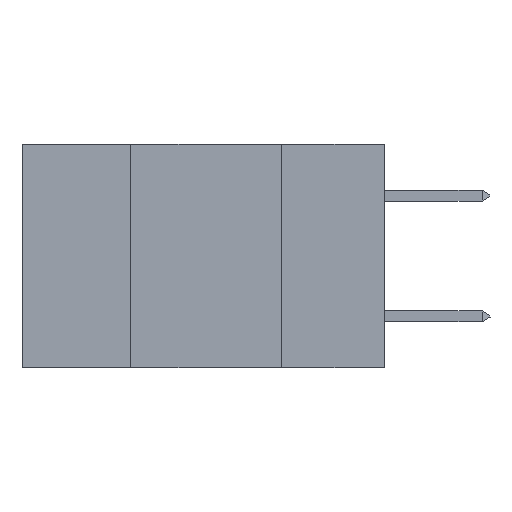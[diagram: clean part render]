
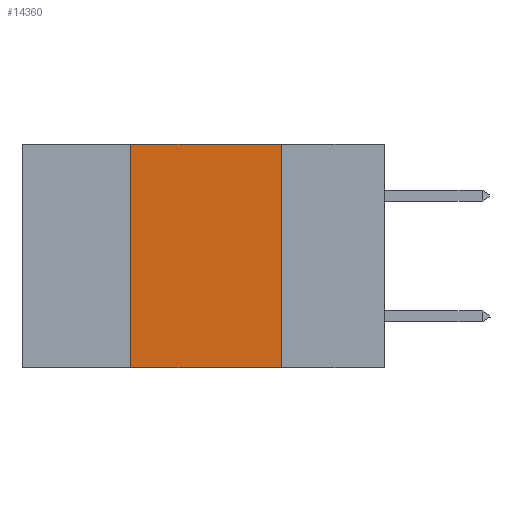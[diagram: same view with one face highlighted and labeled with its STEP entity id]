
A CAD part, left-side view. The second image highlights one B-rep face of the part: STEP entity #14360.
In plain terms, the highlighted planar face has unit normal (-1, 0, 0).
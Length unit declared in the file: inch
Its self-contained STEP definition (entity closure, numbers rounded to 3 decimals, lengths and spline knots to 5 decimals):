
#117 = EDGE_CURVE ( 'NONE', #22170, #18939, #14434, .T. ) ;
#871 = EDGE_CURVE ( 'NONE', #22170, #16552, #5947, .T. ) ;
#1258 = CARTESIAN_POINT ( 'NONE',  ( 0., 0.6, 0. ) ) ;
#1345 = EDGE_LOOP ( 'NONE', ( #12845, #10426, #2112, #11265 ) ) ;
#1416 = CARTESIAN_POINT ( 'NONE',  ( 0., 0.42, -0.37 ) ) ;
#1910 = VECTOR ( 'NONE', #8834, 39.37008 ) ;
#2112 = ORIENTED_EDGE ( 'NONE', *, *, #871, .F. ) ;
#2234 = EDGE_CURVE ( 'NONE', #16552, #11290, #8566, .T. ) ;
#2984 = CARTESIAN_POINT ( 'NONE',  ( 0., 0.42, 0. ) ) ;
#4372 = CARTESIAN_POINT ( 'NONE',  ( 0., 0.17, 0. ) ) ;
#4611 = VECTOR ( 'NONE', #12318, 39.37008 ) ;
#5947 = LINE ( 'NONE', #15566, #21782 ) ;
#7829 = CARTESIAN_POINT ( 'NONE',  ( 0., 0.17, -0.37 ) ) ;
#8566 = LINE ( 'NONE', #12587, #1910 ) ;
#8834 = DIRECTION ( 'NONE',  ( 0., -1., 0. ) ) ;
#9428 = LINE ( 'NONE', #4372, #4611 ) ;
#10426 = ORIENTED_EDGE ( 'NONE', *, *, #2234, .F. ) ;
#11265 = ORIENTED_EDGE ( 'NONE', *, *, #117, .T. ) ;
#11290 = VERTEX_POINT ( 'NONE', #21373 ) ;
#11347 = AXIS2_PLACEMENT_3D ( 'NONE', #1258, #20979, #24919 ) ;
#11934 = DIRECTION ( 'NONE',  ( 0., 0., 1. ) ) ;
#11954 = FACE_OUTER_BOUND ( 'NONE', #1345, .T. ) ;
#12318 = DIRECTION ( 'NONE',  ( 0., 0., -1. ) ) ;
#12587 = CARTESIAN_POINT ( 'NONE',  ( 0., 0.6, 0. ) ) ;
#12590 = PLANE ( 'NONE',  #11347 ) ;
#12845 = ORIENTED_EDGE ( 'NONE', *, *, #16313, .F. ) ;
#14360 = ADVANCED_FACE ( 'NONE', ( #11954 ), #12590, .F. ) ;
#14434 = LINE ( 'NONE', #24531, #18875 ) ;
#15566 = CARTESIAN_POINT ( 'NONE',  ( 0., 0.42, 0. ) ) ;
#16313 = EDGE_CURVE ( 'NONE', #11290, #18939, #9428, .T. ) ;
#16552 = VERTEX_POINT ( 'NONE', #2984 ) ;
#18875 = VECTOR ( 'NONE', #23652, 39.37008 ) ;
#18939 = VERTEX_POINT ( 'NONE', #7829 ) ;
#20979 = DIRECTION ( 'NONE',  ( 1., 0., 0. ) ) ;
#21373 = CARTESIAN_POINT ( 'NONE',  ( 0., 0.17, 0. ) ) ;
#21782 = VECTOR ( 'NONE', #11934, 39.37008 ) ;
#22170 = VERTEX_POINT ( 'NONE', #1416 ) ;
#23652 = DIRECTION ( 'NONE',  ( 0., -1., 0. ) ) ;
#24531 = CARTESIAN_POINT ( 'NONE',  ( 0., 0.6, -0.37 ) ) ;
#24919 = DIRECTION ( 'NONE',  ( 0., 0., -1. ) ) ;
